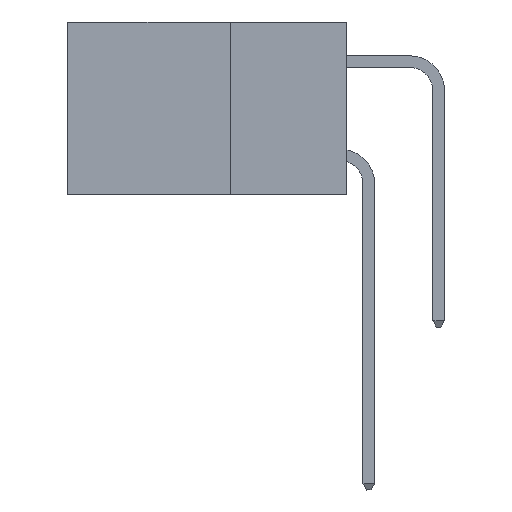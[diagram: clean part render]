
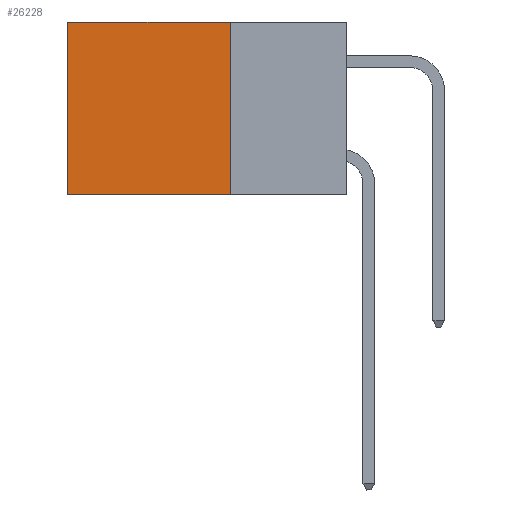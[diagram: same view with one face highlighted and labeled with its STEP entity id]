
A CAD part, left-side view. The second image highlights one B-rep face of the part: STEP entity #26228.
In plain terms, the highlighted planar face has unit normal (-1, 0, 0).
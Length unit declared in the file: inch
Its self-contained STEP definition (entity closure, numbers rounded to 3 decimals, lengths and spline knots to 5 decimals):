
#994 = VERTEX_POINT ( 'NONE', #40519 ) ;
#2808 = ORIENTED_EDGE ( 'NONE', *, *, #32250, .F. ) ;
#4829 = VERTEX_POINT ( 'NONE', #33583 ) ;
#4923 = DIRECTION ( 'NONE',  ( 0., 0., -1. ) ) ;
#5135 = CARTESIAN_POINT ( 'NONE',  ( 0.2875, 0.25, -0.37 ) ) ;
#5630 = ORIENTED_EDGE ( 'NONE', *, *, #6867, .F. ) ;
#6867 = EDGE_CURVE ( 'NONE', #16614, #18503, #24560, .T. ) ;
#6971 = PLANE ( 'NONE',  #42478 ) ;
#7451 = ORIENTED_EDGE ( 'NONE', *, *, #12117, .T. ) ;
#8754 = VECTOR ( 'NONE', #31486, 39.37008 ) ;
#10516 = CARTESIAN_POINT ( 'NONE',  ( 0.2875, 0.25, 0. ) ) ;
#12117 = EDGE_CURVE ( 'NONE', #994, #4829, #39321, .T. ) ;
#12423 = VECTOR ( 'NONE', #4923, 39.37008 ) ;
#13459 = VECTOR ( 'NONE', #26089, 39.37008 ) ;
#14044 = DIRECTION ( 'NONE',  ( 0., 0., -1. ) ) ;
#16584 = CARTESIAN_POINT ( 'NONE',  ( 0.2875, 0.25, -0.37 ) ) ;
#16614 = VERTEX_POINT ( 'NONE', #17058 ) ;
#17058 = CARTESIAN_POINT ( 'NONE',  ( 0.2875, 0.25, 0. ) ) ;
#18503 = VERTEX_POINT ( 'NONE', #16584 ) ;
#22746 = LINE ( 'NONE', #5135, #13459 ) ;
#24560 = LINE ( 'NONE', #32226, #43358 ) ;
#24585 = EDGE_CURVE ( 'NONE', #16614, #994, #27343, .T. ) ;
#26089 = DIRECTION ( 'NONE',  ( 0., 1., 0. ) ) ;
#26228 = ADVANCED_FACE ( 'NONE', ( #29386 ), #6971, .F. ) ;
#27343 = LINE ( 'NONE', #27897, #8754 ) ;
#27897 = CARTESIAN_POINT ( 'NONE',  ( 0.2875, 0.25, 0. ) ) ;
#29386 = FACE_OUTER_BOUND ( 'NONE', #37916, .T. ) ;
#29461 = CARTESIAN_POINT ( 'NONE',  ( 0.2875, 0.6, 0. ) ) ;
#31486 = DIRECTION ( 'NONE',  ( 0., 1., 0. ) ) ;
#32226 = CARTESIAN_POINT ( 'NONE',  ( 0.2875, 0.25, 0. ) ) ;
#32250 = EDGE_CURVE ( 'NONE', #18503, #4829, #22746, .T. ) ;
#33583 = CARTESIAN_POINT ( 'NONE',  ( 0.2875, 0.6, -0.37 ) ) ;
#35052 = DIRECTION ( 'NONE',  ( 1., 0., 0. ) ) ;
#35786 = DIRECTION ( 'NONE',  ( 0., 0., -1. ) ) ;
#37916 = EDGE_LOOP ( 'NONE', ( #7451, #2808, #5630, #45295 ) ) ;
#39321 = LINE ( 'NONE', #29461, #12423 ) ;
#40519 = CARTESIAN_POINT ( 'NONE',  ( 0.2875, 0.6, 0. ) ) ;
#42478 = AXIS2_PLACEMENT_3D ( 'NONE', #10516, #35052, #14044 ) ;
#43358 = VECTOR ( 'NONE', #35786, 39.37008 ) ;
#45295 = ORIENTED_EDGE ( 'NONE', *, *, #24585, .T. ) ;
